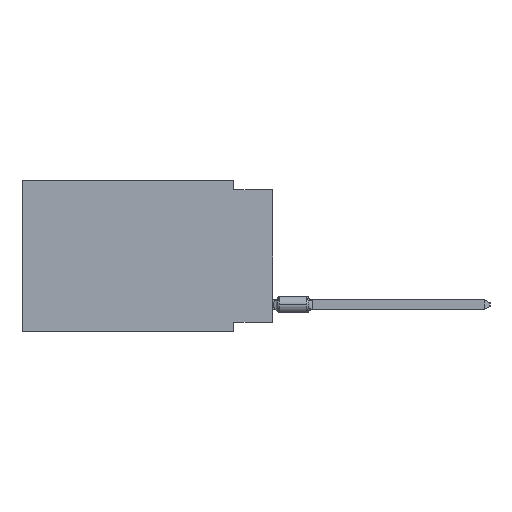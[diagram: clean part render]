
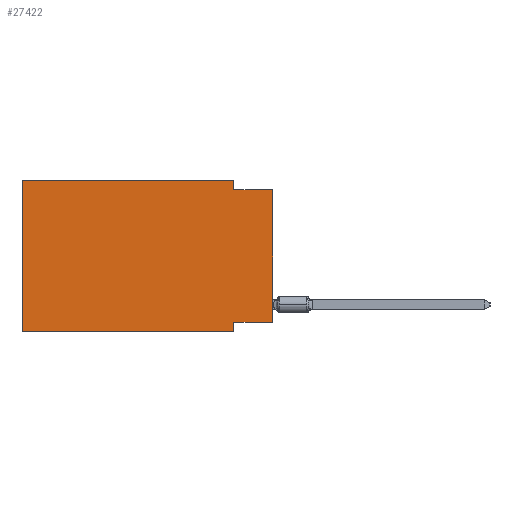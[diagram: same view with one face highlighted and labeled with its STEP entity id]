
A CAD part, left-side view. The second image highlights one B-rep face of the part: STEP entity #27422.
In plain terms, the highlighted planar face has unit normal (-1, 0, 0).
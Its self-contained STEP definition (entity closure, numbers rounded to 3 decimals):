
#303 = ORIENTED_EDGE ( 'NONE', *, *, #75140, .F. ) ;
#1033 = DIRECTION ( 'NONE',  ( 0., 0., -1. ) ) ;
#1793 = EDGE_CURVE ( 'NONE', #38224, #51459, #45871, .T. ) ;
#5000 = EDGE_CURVE ( 'NONE', #65971, #46458, #25578, .T. ) ;
#5319 = DIRECTION ( 'NONE',  ( 0., 0., 1. ) ) ;
#5717 = LINE ( 'NONE', #12394, #48852 ) ;
#6355 = VECTOR ( 'NONE', #47802, 1000. ) ;
#6814 = CARTESIAN_POINT ( 'NONE',  ( 0., 0., 0. ) ) ;
#7775 = CARTESIAN_POINT ( 'NONE',  ( 0., 2.54, -9.906 ) ) ;
#8016 = VECTOR ( 'NONE', #82861, 1000. ) ;
#9034 = VERTEX_POINT ( 'NONE', #65395 ) ;
#9559 = CARTESIAN_POINT ( 'NONE',  ( 0., 16.383, -9.906 ) ) ;
#9942 = ORIENTED_EDGE ( 'NONE', *, *, #78529, .T. ) ;
#10362 = CARTESIAN_POINT ( 'NONE',  ( 0., 2.54, -0.635 ) ) ;
#12170 = LINE ( 'NONE', #6814, #71908 ) ;
#12394 = CARTESIAN_POINT ( 'NONE',  ( 0., 16.383, 0. ) ) ;
#13263 = DIRECTION ( 'NONE',  ( 0., -1., 0. ) ) ;
#14336 = DIRECTION ( 'NONE',  ( 0., 0., -1. ) ) ;
#16966 = EDGE_LOOP ( 'NONE', ( #74789, #44978, #40216, #303, #67074, #9942, #19330, #43571 ) ) ;
#18945 = PLANE ( 'NONE',  #21160 ) ;
#19330 = ORIENTED_EDGE ( 'NONE', *, *, #37473, .F. ) ;
#20606 = LINE ( 'NONE', #67444, #6355 ) ;
#21160 = AXIS2_PLACEMENT_3D ( 'NONE', #46136, #73369, #14336 ) ;
#21187 = VECTOR ( 'NONE', #1033, 1000. ) ;
#21359 = CARTESIAN_POINT ( 'NONE',  ( 0., 0., -9.271 ) ) ;
#22244 = VERTEX_POINT ( 'NONE', #28836 ) ;
#25578 = LINE ( 'NONE', #73299, #67876 ) ;
#25986 = DIRECTION ( 'NONE',  ( 0., 0., 1. ) ) ;
#27339 = DIRECTION ( 'NONE',  ( 0., -1., 0. ) ) ;
#27422 = ADVANCED_FACE ( 'NONE', ( #80033 ), #18945, .F. ) ;
#27706 = DIRECTION ( 'NONE',  ( 0., 0., -1. ) ) ;
#28836 = CARTESIAN_POINT ( 'NONE',  ( 0., 2.54, 0. ) ) ;
#28881 = EDGE_CURVE ( 'NONE', #9034, #46458, #12170, .T. ) ;
#33016 = VECTOR ( 'NONE', #27706, 1000. ) ;
#34380 = LINE ( 'NONE', #69156, #33016 ) ;
#35045 = EDGE_CURVE ( 'NONE', #9034, #57427, #84188, .T. ) ;
#37473 = EDGE_CURVE ( 'NONE', #57427, #39989, #62955, .T. ) ;
#37933 = CARTESIAN_POINT ( 'NONE',  ( 0., 16.383, 0. ) ) ;
#38224 = VERTEX_POINT ( 'NONE', #9559 ) ;
#39989 = VERTEX_POINT ( 'NONE', #7775 ) ;
#40216 = ORIENTED_EDGE ( 'NONE', *, *, #86583, .F. ) ;
#41743 = VECTOR ( 'NONE', #5319, 1000. ) ;
#43571 = ORIENTED_EDGE ( 'NONE', *, *, #35045, .F. ) ;
#44978 = ORIENTED_EDGE ( 'NONE', *, *, #5000, .F. ) ;
#45871 = LINE ( 'NONE', #47615, #41743 ) ;
#46136 = CARTESIAN_POINT ( 'NONE',  ( 0., 16.383, 0. ) ) ;
#46458 = VERTEX_POINT ( 'NONE', #54670 ) ;
#47615 = CARTESIAN_POINT ( 'NONE',  ( 0., 16.383, 0. ) ) ;
#47802 = DIRECTION ( 'NONE',  ( 0., -1., 0. ) ) ;
#48852 = VECTOR ( 'NONE', #13263, 1000. ) ;
#49120 = CARTESIAN_POINT ( 'NONE',  ( 0., 2.54, -9.906 ) ) ;
#51459 = VERTEX_POINT ( 'NONE', #37933 ) ;
#54670 = CARTESIAN_POINT ( 'NONE',  ( 0., 0., -0.635 ) ) ;
#57427 = VERTEX_POINT ( 'NONE', #86313 ) ;
#62955 = LINE ( 'NONE', #49120, #21187 ) ;
#65395 = CARTESIAN_POINT ( 'NONE',  ( 0., 0., -9.271 ) ) ;
#65971 = VERTEX_POINT ( 'NONE', #10362 ) ;
#67074 = ORIENTED_EDGE ( 'NONE', *, *, #1793, .F. ) ;
#67444 = CARTESIAN_POINT ( 'NONE',  ( 0., 16.383, -9.906 ) ) ;
#67876 = VECTOR ( 'NONE', #27339, 1000. ) ;
#69156 = CARTESIAN_POINT ( 'NONE',  ( 0., 2.54, 0. ) ) ;
#71908 = VECTOR ( 'NONE', #25986, 1000. ) ;
#73299 = CARTESIAN_POINT ( 'NONE',  ( 0., 0., -0.635 ) ) ;
#73369 = DIRECTION ( 'NONE',  ( 1., 0., 0. ) ) ;
#74789 = ORIENTED_EDGE ( 'NONE', *, *, #28881, .T. ) ;
#75140 = EDGE_CURVE ( 'NONE', #51459, #22244, #5717, .T. ) ;
#78529 = EDGE_CURVE ( 'NONE', #38224, #39989, #20606, .T. ) ;
#80033 = FACE_OUTER_BOUND ( 'NONE', #16966, .T. ) ;
#82861 = DIRECTION ( 'NONE',  ( 0., 1., 0. ) ) ;
#84188 = LINE ( 'NONE', #21359, #8016 ) ;
#86313 = CARTESIAN_POINT ( 'NONE',  ( 0., 2.54, -9.271 ) ) ;
#86583 = EDGE_CURVE ( 'NONE', #22244, #65971, #34380, .T. ) ;
